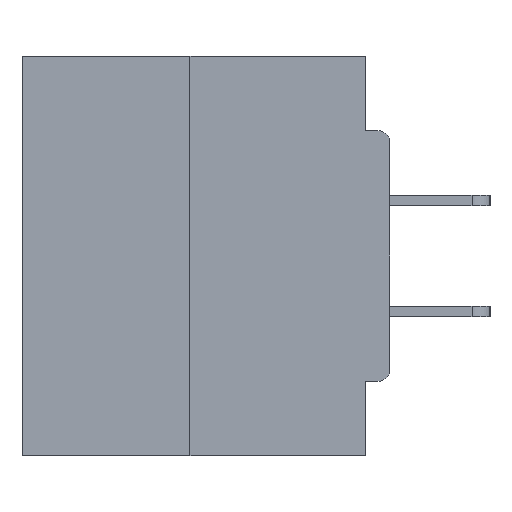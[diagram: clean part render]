
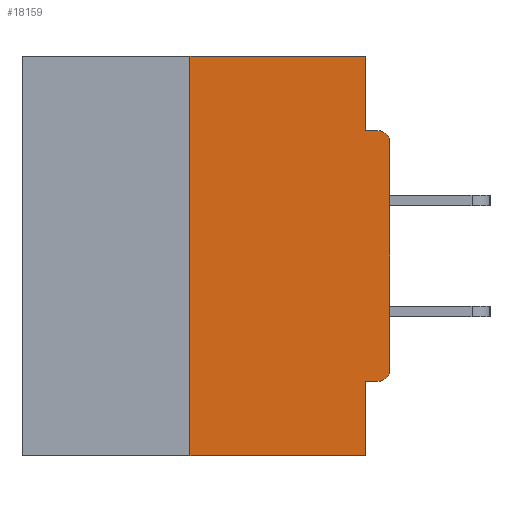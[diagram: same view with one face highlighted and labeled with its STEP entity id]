
A CAD part, left-side view. The second image highlights one B-rep face of the part: STEP entity #18159.
In plain terms, the highlighted planar face has unit normal (-1, 0, 0).
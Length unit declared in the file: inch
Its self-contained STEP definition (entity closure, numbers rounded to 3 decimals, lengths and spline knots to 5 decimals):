
#25 = LINE ( 'NONE', #5553, #16231 ) ;
#305 = CARTESIAN_POINT ( 'NONE',  ( 0., 0.015, -0.3915 ) ) ;
#782 = ORIENTED_EDGE ( 'NONE', *, *, #24443, .T. ) ;
#1273 = CARTESIAN_POINT ( 'NONE',  ( 0., 0., -0.1085 ) ) ;
#1465 = DIRECTION ( 'NONE',  ( -1., 0., 0. ) ) ;
#1719 = CARTESIAN_POINT ( 'NONE',  ( 0., 0.46, -0.5 ) ) ;
#1842 = AXIS2_PLACEMENT_3D ( 'NONE', #21308, #26258, #21653 ) ;
#2194 = CARTESIAN_POINT ( 'NONE',  ( 0., 0.031, -0.5 ) ) ;
#2805 = LINE ( 'NONE', #24099, #23181 ) ;
#2935 = ORIENTED_EDGE ( 'NONE', *, *, #29014, .T. ) ;
#3096 = EDGE_CURVE ( 'NONE', #12006, #22850, #14382, .T. ) ;
#4182 = DIRECTION ( 'NONE',  ( 0., -1., 0. ) ) ;
#4881 = CARTESIAN_POINT ( 'NONE',  ( 0., 0.46, 0. ) ) ;
#5553 = CARTESIAN_POINT ( 'NONE',  ( 0., 0.031, -0.5 ) ) ;
#6035 = CARTESIAN_POINT ( 'NONE',  ( 0., 0.031, 0. ) ) ;
#6052 = FACE_OUTER_BOUND ( 'NONE', #27659, .T. ) ;
#6265 = VERTEX_POINT ( 'NONE', #15883 ) ;
#7038 = LINE ( 'NONE', #25696, #12064 ) ;
#7157 = EDGE_CURVE ( 'NONE', #6265, #19683, #13409, .T. ) ;
#7850 = VERTEX_POINT ( 'NONE', #9512 ) ;
#9512 = CARTESIAN_POINT ( 'NONE',  ( 0., 0.25, -0.5 ) ) ;
#9608 = DIRECTION ( 'NONE',  ( 0., -1., 0. ) ) ;
#9695 = DIRECTION ( 'NONE',  ( 0., -1., 0. ) ) ;
#10278 = LINE ( 'NONE', #30031, #16456 ) ;
#10350 = DIRECTION ( 'NONE',  ( -1., 0., 0. ) ) ;
#10922 = VECTOR ( 'NONE', #4182, 39.37008 ) ;
#12006 = VERTEX_POINT ( 'NONE', #15211 ) ;
#12034 = CARTESIAN_POINT ( 'NONE',  ( 0., 0.015, -0.0935 ) ) ;
#12064 = VECTOR ( 'NONE', #13593, 39.37008 ) ;
#12475 = CARTESIAN_POINT ( 'NONE',  ( 0., 0.015, -0.4065 ) ) ;
#12502 = LINE ( 'NONE', #1719, #10922 ) ;
#12834 = DIRECTION ( 'NONE',  ( 0., 0., -1. ) ) ;
#12879 = ORIENTED_EDGE ( 'NONE', *, *, #16266, .T. ) ;
#13409 = LINE ( 'NONE', #4881, #31100 ) ;
#13488 = DIRECTION ( 'NONE',  ( 0., 0., -1. ) ) ;
#13593 = DIRECTION ( 'NONE',  ( 0., 1., 0. ) ) ;
#14382 = LINE ( 'NONE', #22068, #15514 ) ;
#14812 = AXIS2_PLACEMENT_3D ( 'NONE', #305, #10350, #12834 ) ;
#14992 = VERTEX_POINT ( 'NONE', #1273 ) ;
#15211 = CARTESIAN_POINT ( 'NONE',  ( 0., 0.031, -0.0935 ) ) ;
#15426 = EDGE_CURVE ( 'NONE', #7850, #26910, #12502, .T. ) ;
#15514 = VECTOR ( 'NONE', #9608, 39.37008 ) ;
#15876 = EDGE_CURVE ( 'NONE', #23130, #25853, #7038, .T. ) ;
#15883 = CARTESIAN_POINT ( 'NONE',  ( 0., 0.25, 0. ) ) ;
#16231 = VECTOR ( 'NONE', #18303, 39.37008 ) ;
#16243 = DIRECTION ( 'NONE',  ( 0., 0., -1. ) ) ;
#16266 = EDGE_CURVE ( 'NONE', #14992, #22850, #27382, .T. ) ;
#16456 = VECTOR ( 'NONE', #27233, 39.37008 ) ;
#16920 = DIRECTION ( 'NONE',  ( 0., 0., 1. ) ) ;
#17552 = ORIENTED_EDGE ( 'NONE', *, *, #24511, .F. ) ;
#17554 = VECTOR ( 'NONE', #13488, 39.37008 ) ;
#17905 = ORIENTED_EDGE ( 'NONE', *, *, #7157, .F. ) ;
#18159 = ADVANCED_FACE ( 'NONE', ( #6052 ), #19188, .F. ) ;
#18303 = DIRECTION ( 'NONE',  ( 0., 0., -1. ) ) ;
#18982 = ORIENTED_EDGE ( 'NONE', *, *, #15876, .F. ) ;
#19188 = PLANE ( 'NONE',  #1842 ) ;
#19683 = VERTEX_POINT ( 'NONE', #6035 ) ;
#21291 = ORIENTED_EDGE ( 'NONE', *, *, #15426, .T. ) ;
#21308 = CARTESIAN_POINT ( 'NONE',  ( 0., 0.46, 0. ) ) ;
#21436 = ORIENTED_EDGE ( 'NONE', *, *, #30326, .F. ) ;
#21653 = DIRECTION ( 'NONE',  ( 0., 0., -1. ) ) ;
#22068 = CARTESIAN_POINT ( 'NONE',  ( 0., 0., -0.0935 ) ) ;
#22427 = VERTEX_POINT ( 'NONE', #30226 ) ;
#22850 = VERTEX_POINT ( 'NONE', #12034 ) ;
#23130 = VERTEX_POINT ( 'NONE', #12475 ) ;
#23181 = VECTOR ( 'NONE', #16920, 39.37008 ) ;
#23260 = LINE ( 'NONE', #28056, #17554 ) ;
#23586 = EDGE_CURVE ( 'NONE', #7850, #6265, #2805, .T. ) ;
#24099 = CARTESIAN_POINT ( 'NONE',  ( 0., 0.25, 0. ) ) ;
#24443 = EDGE_CURVE ( 'NONE', #23130, #22427, #26625, .T. ) ;
#24511 = EDGE_CURVE ( 'NONE', #25853, #26910, #25, .T. ) ;
#25696 = CARTESIAN_POINT ( 'NONE',  ( 0., 0., -0.4065 ) ) ;
#25853 = VERTEX_POINT ( 'NONE', #30967 ) ;
#26258 = DIRECTION ( 'NONE',  ( 1., 0., 0. ) ) ;
#26625 = CIRCLE ( 'NONE', #14812, 0.015 ) ;
#26810 = ORIENTED_EDGE ( 'NONE', *, *, #3096, .F. ) ;
#26910 = VERTEX_POINT ( 'NONE', #2194 ) ;
#27233 = DIRECTION ( 'NONE',  ( 0., 0., 1. ) ) ;
#27382 = CIRCLE ( 'NONE', #28789, 0.015 ) ;
#27659 = EDGE_LOOP ( 'NONE', ( #17905, #29555, #21291, #17552, #18982, #782, #2935, #12879, #26810, #21436 ) ) ;
#28056 = CARTESIAN_POINT ( 'NONE',  ( 0., 0.031, 0. ) ) ;
#28146 = CARTESIAN_POINT ( 'NONE',  ( 0., 0.015, -0.1085 ) ) ;
#28789 = AXIS2_PLACEMENT_3D ( 'NONE', #28146, #1465, #16243 ) ;
#29014 = EDGE_CURVE ( 'NONE', #22427, #14992, #10278, .T. ) ;
#29555 = ORIENTED_EDGE ( 'NONE', *, *, #23586, .F. ) ;
#30031 = CARTESIAN_POINT ( 'NONE',  ( 0., 0., 0. ) ) ;
#30226 = CARTESIAN_POINT ( 'NONE',  ( 0., 0., -0.3915 ) ) ;
#30326 = EDGE_CURVE ( 'NONE', #19683, #12006, #23260, .T. ) ;
#30967 = CARTESIAN_POINT ( 'NONE',  ( 0., 0.031, -0.4065 ) ) ;
#31100 = VECTOR ( 'NONE', #9695, 39.37008 ) ;
